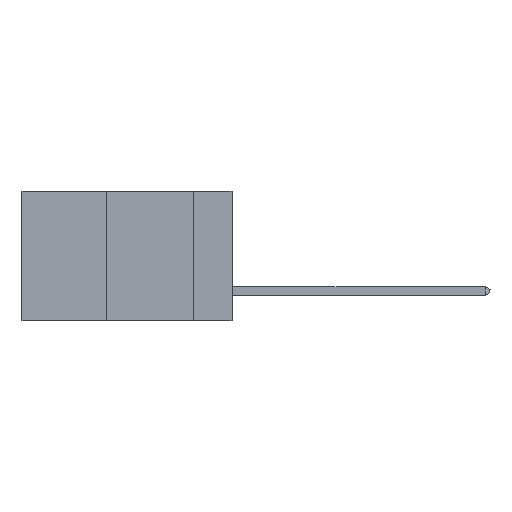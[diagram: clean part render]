
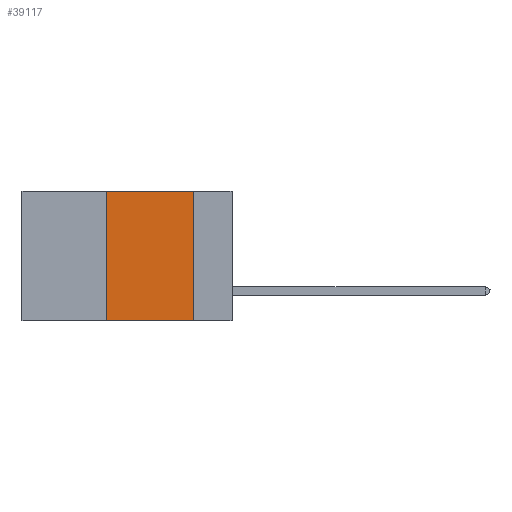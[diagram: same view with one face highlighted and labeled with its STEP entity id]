
A CAD part, left-side view. The second image highlights one B-rep face of the part: STEP entity #39117.
In plain terms, the highlighted planar face has unit normal (-1, 0, 0).
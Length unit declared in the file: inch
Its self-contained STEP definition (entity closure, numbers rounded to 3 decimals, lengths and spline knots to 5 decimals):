
#1653 = LINE ( 'NONE', #17192, #38942 ) ;
#2830 = CARTESIAN_POINT ( 'NONE',  ( 0., 0.11, 0. ) ) ;
#3920 = VERTEX_POINT ( 'NONE', #5844 ) ;
#5672 = VERTEX_POINT ( 'NONE', #27794 ) ;
#5844 = CARTESIAN_POINT ( 'NONE',  ( 0., 0.11, 0. ) ) ;
#6404 = ORIENTED_EDGE ( 'NONE', *, *, #12447, .F. ) ;
#6644 = DIRECTION ( 'NONE',  ( 0., 0., 1. ) ) ;
#8386 = DIRECTION ( 'NONE',  ( 0., -1., 0. ) ) ;
#9129 = LINE ( 'NONE', #17371, #35403 ) ;
#9963 = CARTESIAN_POINT ( 'NONE',  ( 0., 0.6, 0. ) ) ;
#11619 = CARTESIAN_POINT ( 'NONE',  ( 0., 0.6, 0. ) ) ;
#12447 = EDGE_CURVE ( 'NONE', #20761, #23234, #9129, .T. ) ;
#16083 = DIRECTION ( 'NONE',  ( 0., 0., -1. ) ) ;
#17192 = CARTESIAN_POINT ( 'NONE',  ( 0., 0.6, -0.37 ) ) ;
#17371 = CARTESIAN_POINT ( 'NONE',  ( 0., 0.36, 0. ) ) ;
#19030 = PLANE ( 'NONE',  #38274 ) ;
#19625 = VECTOR ( 'NONE', #29810, 39.37008 ) ;
#20699 = CARTESIAN_POINT ( 'NONE',  ( 0., 0.36, -0.37 ) ) ;
#20761 = VERTEX_POINT ( 'NONE', #20699 ) ;
#21479 = EDGE_LOOP ( 'NONE', ( #22910, #34750, #6404, #23545 ) ) ;
#21888 = VECTOR ( 'NONE', #32958, 39.37008 ) ;
#22910 = ORIENTED_EDGE ( 'NONE', *, *, #24566, .F. ) ;
#23234 = VERTEX_POINT ( 'NONE', #37451 ) ;
#23545 = ORIENTED_EDGE ( 'NONE', *, *, #36674, .T. ) ;
#24566 = EDGE_CURVE ( 'NONE', #3920, #5672, #33014, .T. ) ;
#25217 = DIRECTION ( 'NONE',  ( 1., 0., 0. ) ) ;
#27794 = CARTESIAN_POINT ( 'NONE',  ( 0., 0.11, -0.37 ) ) ;
#29609 = FACE_OUTER_BOUND ( 'NONE', #21479, .T. ) ;
#29810 = DIRECTION ( 'NONE',  ( 0., 0., -1. ) ) ;
#30540 = EDGE_CURVE ( 'NONE', #23234, #3920, #31920, .T. ) ;
#31920 = LINE ( 'NONE', #11619, #21888 ) ;
#32958 = DIRECTION ( 'NONE',  ( 0., -1., 0. ) ) ;
#33014 = LINE ( 'NONE', #2830, #19625 ) ;
#34750 = ORIENTED_EDGE ( 'NONE', *, *, #30540, .F. ) ;
#35403 = VECTOR ( 'NONE', #6644, 39.37008 ) ;
#36674 = EDGE_CURVE ( 'NONE', #20761, #5672, #1653, .T. ) ;
#37451 = CARTESIAN_POINT ( 'NONE',  ( 0., 0.36, 0. ) ) ;
#38274 = AXIS2_PLACEMENT_3D ( 'NONE', #9963, #25217, #16083 ) ;
#38942 = VECTOR ( 'NONE', #8386, 39.37008 ) ;
#39117 = ADVANCED_FACE ( 'NONE', ( #29609 ), #19030, .F. ) ;
